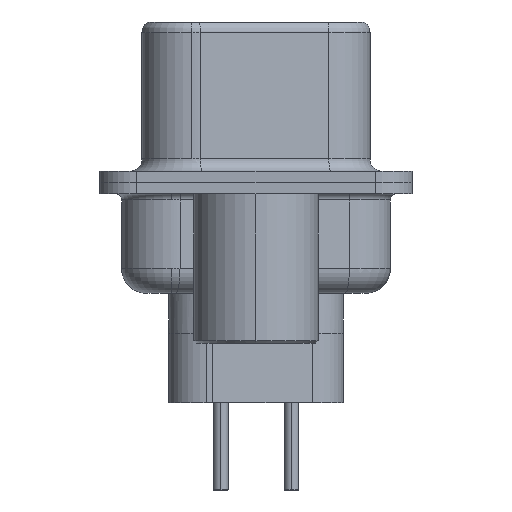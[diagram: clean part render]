
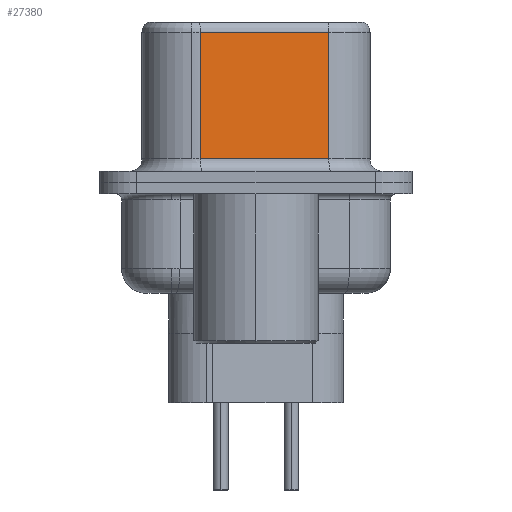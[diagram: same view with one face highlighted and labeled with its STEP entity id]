
A CAD part, left-side view. The second image highlights one B-rep face of the part: STEP entity #27380.
In plain terms, the highlighted planar face has unit normal (-0.985, -0.174, 0).
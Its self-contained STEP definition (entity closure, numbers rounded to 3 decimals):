
#98 = CARTESIAN_POINT ( 'NONE',  ( 4.58, -2.927, 0.95 ) ) ;
#218 = AXIS2_PLACEMENT_3D ( 'NONE', #27152, #7844, #25028 ) ;
#648 = EDGE_CURVE ( 'NONE', #9514, #26753, #19306, .T. ) ;
#4468 = LINE ( 'NONE', #15476, #21166 ) ;
#7340 = CARTESIAN_POINT ( 'NONE',  ( 4.58, -2.927, 6.52 ) ) ;
#7448 = EDGE_CURVE ( 'NONE', #13747, #20031, #10976, .T. ) ;
#7520 = EDGE_CURVE ( 'NONE', #26753, #13747, #4468, .T. ) ;
#7844 = DIRECTION ( 'NONE',  ( 0.985, 0.174, 0. ) ) ;
#8872 = DIRECTION ( 'NONE',  ( 0., 0., -1. ) ) ;
#9514 = VERTEX_POINT ( 'NONE', #21729 ) ;
#10976 = LINE ( 'NONE', #98, #11736 ) ;
#11736 = VECTOR ( 'NONE', #26048, 1000. ) ;
#13154 = ORIENTED_EDGE ( 'NONE', *, *, #22107, .F. ) ;
#13747 = VERTEX_POINT ( 'NONE', #15904 ) ;
#14321 = FACE_OUTER_BOUND ( 'NONE', #15001, .T. ) ;
#14766 = CARTESIAN_POINT ( 'NONE',  ( 3.67, 2.233, 6.02 ) ) ;
#15001 = EDGE_LOOP ( 'NONE', ( #13154, #17520, #17570, #24356 ) ) ;
#15476 = CARTESIAN_POINT ( 'NONE',  ( 3.67, 2.233, 6.52 ) ) ;
#15904 = CARTESIAN_POINT ( 'NONE',  ( 3.67, 2.233, 0.95 ) ) ;
#17520 = ORIENTED_EDGE ( 'NONE', *, *, #648, .T. ) ;
#17570 = ORIENTED_EDGE ( 'NONE', *, *, #7520, .T. ) ;
#18546 = PLANE ( 'NONE',  #218 ) ;
#18736 = VECTOR ( 'NONE', #22562, 1000. ) ;
#19154 = VECTOR ( 'NONE', #21550, 1000. ) ;
#19306 = LINE ( 'NONE', #23675, #19154 ) ;
#20031 = VERTEX_POINT ( 'NONE', #22616 ) ;
#21166 = VECTOR ( 'NONE', #8872, 1000. ) ;
#21550 = DIRECTION ( 'NONE',  ( -0.174, 0.985, 0. ) ) ;
#21729 = CARTESIAN_POINT ( 'NONE',  ( 4.58, -2.927, 6.02 ) ) ;
#22107 = EDGE_CURVE ( 'NONE', #9514, #20031, #24807, .T. ) ;
#22562 = DIRECTION ( 'NONE',  ( 0., 0., -1. ) ) ;
#22616 = CARTESIAN_POINT ( 'NONE',  ( 4.58, -2.927, 0.95 ) ) ;
#23675 = CARTESIAN_POINT ( 'NONE',  ( 4.58, -2.927, 6.02 ) ) ;
#24356 = ORIENTED_EDGE ( 'NONE', *, *, #7448, .T. ) ;
#24807 = LINE ( 'NONE', #7340, #18736 ) ;
#25028 = DIRECTION ( 'NONE',  ( -0.174, 0.985, 0. ) ) ;
#26048 = DIRECTION ( 'NONE',  ( 0.174, -0.985, 0. ) ) ;
#26753 = VERTEX_POINT ( 'NONE', #14766 ) ;
#27152 = CARTESIAN_POINT ( 'NONE',  ( 4.58, -2.927, 6.52 ) ) ;
#27380 = ADVANCED_FACE ( 'NONE', ( #14321 ), #18546, .F. ) ;
